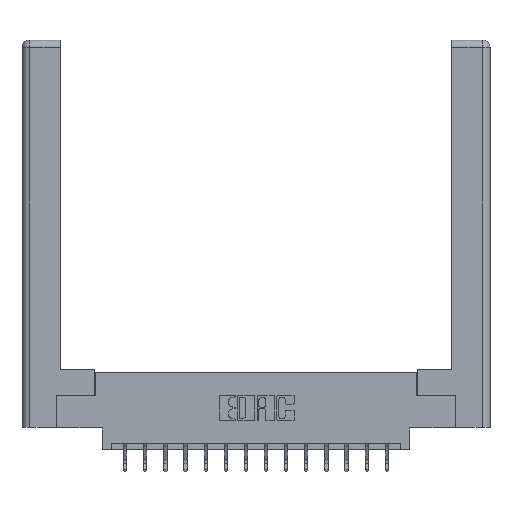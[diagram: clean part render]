
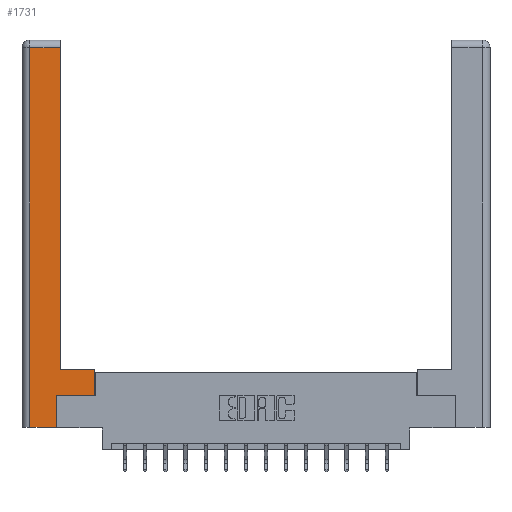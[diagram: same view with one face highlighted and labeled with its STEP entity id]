
A CAD part, top view. The second image highlights one B-rep face of the part: STEP entity #1731.
In plain terms, the highlighted planar face has unit normal (0, 0, 1).
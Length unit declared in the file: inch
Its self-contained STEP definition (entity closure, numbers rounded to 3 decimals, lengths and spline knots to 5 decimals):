
#325 = ORIENTED_EDGE ( 'NONE', *, *, #6913, .T. ) ;
#553 = DIRECTION ( 'NONE',  ( 1., 0., 0. ) ) ;
#764 = VERTEX_POINT ( 'NONE', #12197 ) ;
#853 = VECTOR ( 'NONE', #3279, 39.37008 ) ;
#1416 = CARTESIAN_POINT ( 'NONE',  ( 0.295, 0.45, 0. ) ) ;
#1695 = CARTESIAN_POINT ( 'NONE',  ( 0.565, 0.45, 0. ) ) ;
#1731 = ADVANCED_FACE ( 'NONE', ( #5277 ), #8391, .F. ) ;
#1817 = VECTOR ( 'NONE', #11805, 39.37008 ) ;
#2061 = AXIS2_PLACEMENT_3D ( 'NONE', #2857, #5559, #5735 ) ;
#2248 = LINE ( 'NONE', #16483, #15353 ) ;
#2356 = CARTESIAN_POINT ( 'NONE',  ( 0.0615, 2.94, 0. ) ) ;
#2490 = VECTOR ( 'NONE', #553, 39.37008 ) ;
#2575 = VERTEX_POINT ( 'NONE', #8418 ) ;
#2711 = EDGE_CURVE ( 'NONE', #13711, #2575, #5447, .T. ) ;
#2851 = EDGE_CURVE ( 'NONE', #764, #13711, #7346, .T. ) ;
#2857 = CARTESIAN_POINT ( 'NONE',  ( 0., 0., 0. ) ) ;
#3279 = DIRECTION ( 'NONE',  ( 0., 1., 0. ) ) ;
#3726 = CARTESIAN_POINT ( 'NONE',  ( 0.295, 3., 0. ) ) ;
#3972 = CARTESIAN_POINT ( 'NONE',  ( 0.565, 0.245, 0. ) ) ;
#5077 = DIRECTION ( 'NONE',  ( 0., 1., 0. ) ) ;
#5277 = FACE_OUTER_BOUND ( 'NONE', #13021, .T. ) ;
#5365 = VERTEX_POINT ( 'NONE', #3972 ) ;
#5447 = LINE ( 'NONE', #3726, #13096 ) ;
#5521 = VERTEX_POINT ( 'NONE', #8615 ) ;
#5540 = DIRECTION ( 'NONE',  ( -1., 0., 0. ) ) ;
#5559 = DIRECTION ( 'NONE',  ( 0., 0., -1. ) ) ;
#5709 = LINE ( 'NONE', #7374, #853 ) ;
#5735 = DIRECTION ( 'NONE',  ( -1., 0., 0. ) ) ;
#5766 = DIRECTION ( 'NONE',  ( 0., 1., 0. ) ) ;
#6913 = EDGE_CURVE ( 'NONE', #2575, #7754, #8775, .T. ) ;
#7154 = LINE ( 'NONE', #16541, #8641 ) ;
#7179 = ORIENTED_EDGE ( 'NONE', *, *, #2711, .T. ) ;
#7346 = LINE ( 'NONE', #1416, #16437 ) ;
#7362 = VECTOR ( 'NONE', #5766, 39.37008 ) ;
#7374 = CARTESIAN_POINT ( 'NONE',  ( 0.265, 0.245, 0. ) ) ;
#7754 = VERTEX_POINT ( 'NONE', #15655 ) ;
#8391 = PLANE ( 'NONE',  #2061 ) ;
#8418 = CARTESIAN_POINT ( 'NONE',  ( 0.295, 2.94, 0. ) ) ;
#8615 = CARTESIAN_POINT ( 'NONE',  ( 0.0615, 0., 0. ) ) ;
#8641 = VECTOR ( 'NONE', #13668, 39.37008 ) ;
#8728 = CARTESIAN_POINT ( 'NONE',  ( 0.265, 0., 0. ) ) ;
#8775 = LINE ( 'NONE', #2356, #1817 ) ;
#9966 = EDGE_CURVE ( 'NONE', #13375, #17462, #5709, .T. ) ;
#10710 = LINE ( 'NONE', #16832, #2490 ) ;
#11300 = CARTESIAN_POINT ( 'NONE',  ( 0.265, 0.245, 0. ) ) ;
#11405 = LINE ( 'NONE', #1695, #7362 ) ;
#11515 = CARTESIAN_POINT ( 'NONE',  ( 0.295, 0.45, 0. ) ) ;
#11590 = EDGE_CURVE ( 'NONE', #17462, #5365, #10710, .T. ) ;
#11805 = DIRECTION ( 'NONE',  ( -1., 0., 0. ) ) ;
#11904 = ORIENTED_EDGE ( 'NONE', *, *, #15995, .T. ) ;
#12197 = CARTESIAN_POINT ( 'NONE',  ( 0.565, 0.45, 0. ) ) ;
#12770 = ORIENTED_EDGE ( 'NONE', *, *, #2851, .T. ) ;
#13021 = EDGE_LOOP ( 'NONE', ( #7179, #325, #11904, #16192, #16850, #15251, #16132, #12770 ) ) ;
#13096 = VECTOR ( 'NONE', #5077, 39.37008 ) ;
#13375 = VERTEX_POINT ( 'NONE', #8728 ) ;
#13668 = DIRECTION ( 'NONE',  ( 0., -1., 0. ) ) ;
#13711 = VERTEX_POINT ( 'NONE', #11515 ) ;
#15251 = ORIENTED_EDGE ( 'NONE', *, *, #11590, .T. ) ;
#15303 = DIRECTION ( 'NONE',  ( 1., 0., 0. ) ) ;
#15353 = VECTOR ( 'NONE', #15303, 39.37008 ) ;
#15655 = CARTESIAN_POINT ( 'NONE',  ( 0.0615, 2.94, 0. ) ) ;
#15892 = EDGE_CURVE ( 'NONE', #5365, #764, #11405, .T. ) ;
#15995 = EDGE_CURVE ( 'NONE', #7754, #5521, #7154, .T. ) ;
#16132 = ORIENTED_EDGE ( 'NONE', *, *, #15892, .T. ) ;
#16192 = ORIENTED_EDGE ( 'NONE', *, *, #17194, .T. ) ;
#16437 = VECTOR ( 'NONE', #5540, 39.37008 ) ;
#16483 = CARTESIAN_POINT ( 'NONE',  ( 0.265, 0., 0. ) ) ;
#16541 = CARTESIAN_POINT ( 'NONE',  ( 0.0615, 0., 0. ) ) ;
#16832 = CARTESIAN_POINT ( 'NONE',  ( 0.565, 0.245, 0. ) ) ;
#16850 = ORIENTED_EDGE ( 'NONE', *, *, #9966, .T. ) ;
#17194 = EDGE_CURVE ( 'NONE', #5521, #13375, #2248, .T. ) ;
#17462 = VERTEX_POINT ( 'NONE', #11300 ) ;
